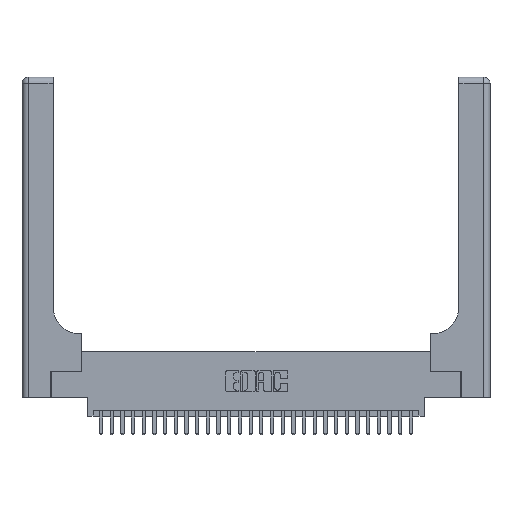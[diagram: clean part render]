
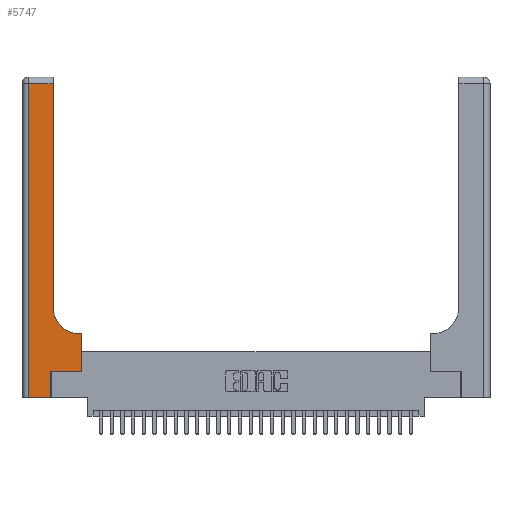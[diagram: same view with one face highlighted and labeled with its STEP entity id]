
A CAD part, top view. The second image highlights one B-rep face of the part: STEP entity #5747.
In plain terms, the highlighted planar face has unit normal (0, 0, 1).
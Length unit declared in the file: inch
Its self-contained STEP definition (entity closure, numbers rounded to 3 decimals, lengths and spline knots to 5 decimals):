
#76 = FACE_OUTER_BOUND ( 'NONE', #607, .T. ) ;
#607 = EDGE_LOOP ( 'NONE', ( #3816, #5903, #7704, #10408, #11895, #14027, #17095, #24863, #25956 ) ) ;
#876 = LINE ( 'NONE', #13336, #19120 ) ;
#1017 = CARTESIAN_POINT ( 'NONE',  ( 0.2915, 0.6, 0.37 ) ) ;
#1021 = CARTESIAN_POINT ( 'NONE',  ( 0.5415, 0.85, 0.37 ) ) ;
#1542 = LINE ( 'NONE', #1017, #4173 ) ;
#2059 = CARTESIAN_POINT ( 'NONE',  ( 0.5585, 0.6, 0.37 ) ) ;
#2779 = CARTESIAN_POINT ( 'NONE',  ( 0., 3., 0.37 ) ) ;
#3364 = LINE ( 'NONE', #28676, #16744 ) ;
#3437 = DIRECTION ( 'NONE',  ( 1., 0., 0. ) ) ;
#3473 = EDGE_CURVE ( 'NONE', #10679, #6550, #18507, .T. ) ;
#3590 = VERTEX_POINT ( 'NONE', #25736 ) ;
#3816 = ORIENTED_EDGE ( 'NONE', *, *, #27646, .T. ) ;
#4173 = VECTOR ( 'NONE', #24649, 39.37008 ) ;
#4844 = DIRECTION ( 'NONE',  ( -1., 0., 0. ) ) ;
#5107 = VECTOR ( 'NONE', #30121, 39.37008 ) ;
#5191 = DIRECTION ( 'NONE',  ( 0., 0., -1. ) ) ;
#5558 = VERTEX_POINT ( 'NONE', #2059 ) ;
#5747 = ADVANCED_FACE ( 'NONE', ( #76 ), #17042, .F. ) ;
#5893 = CARTESIAN_POINT ( 'NONE',  ( 0.06, 3., 0.37 ) ) ;
#5903 = ORIENTED_EDGE ( 'NONE', *, *, #14313, .T. ) ;
#6550 = VERTEX_POINT ( 'NONE', #22032 ) ;
#7219 = CARTESIAN_POINT ( 'NONE',  ( 0., 2.94, 0.37 ) ) ;
#7704 = ORIENTED_EDGE ( 'NONE', *, *, #7929, .T. ) ;
#7929 = EDGE_CURVE ( 'NONE', #3590, #10679, #9997, .T. ) ;
#8371 = LINE ( 'NONE', #11096, #13962 ) ;
#8708 = DIRECTION ( 'NONE',  ( 0., 1., 0. ) ) ;
#8844 = VERTEX_POINT ( 'NONE', #20648 ) ;
#9689 = VERTEX_POINT ( 'NONE', #12476 ) ;
#9997 = LINE ( 'NONE', #5893, #17112 ) ;
#10406 = VECTOR ( 'NONE', #26444, 39.37008 ) ;
#10408 = ORIENTED_EDGE ( 'NONE', *, *, #3473, .T. ) ;
#10679 = VERTEX_POINT ( 'NONE', #15997 ) ;
#10948 = DIRECTION ( 'NONE',  ( 1., 0., 0. ) ) ;
#11096 = CARTESIAN_POINT ( 'NONE',  ( 0.5585, 0.25, 0.37 ) ) ;
#11895 = ORIENTED_EDGE ( 'NONE', *, *, #12980, .T. ) ;
#12476 = CARTESIAN_POINT ( 'NONE',  ( 0.269, 0.25, 0.37 ) ) ;
#12980 = EDGE_CURVE ( 'NONE', #6550, #9689, #3364, .T. ) ;
#13336 = CARTESIAN_POINT ( 'NONE',  ( 0.269, 0.25, 0.37 ) ) ;
#13962 = VECTOR ( 'NONE', #8708, 39.37008 ) ;
#14027 = ORIENTED_EDGE ( 'NONE', *, *, #29361, .T. ) ;
#14313 = EDGE_CURVE ( 'NONE', #8844, #3590, #17438, .T. ) ;
#14618 = CARTESIAN_POINT ( 'NONE',  ( 0.2915, 3., 0.37 ) ) ;
#14659 = CARTESIAN_POINT ( 'NONE',  ( 0.5585, 0.25, 0.37 ) ) ;
#15997 = CARTESIAN_POINT ( 'NONE',  ( 0.06, 0., 0.37 ) ) ;
#16744 = VECTOR ( 'NONE', #26422, 39.37008 ) ;
#16760 = LINE ( 'NONE', #14618, #10406 ) ;
#17042 = PLANE ( 'NONE',  #22698 ) ;
#17095 = ORIENTED_EDGE ( 'NONE', *, *, #18172, .T. ) ;
#17112 = VECTOR ( 'NONE', #20122, 39.37008 ) ;
#17438 = LINE ( 'NONE', #7219, #29125 ) ;
#17695 = DIRECTION ( 'NONE',  ( 0., 0., -1. ) ) ;
#18172 = EDGE_CURVE ( 'NONE', #27009, #5558, #8371, .T. ) ;
#18385 = CARTESIAN_POINT ( 'NONE',  ( 0., 0., 0.37 ) ) ;
#18507 = LINE ( 'NONE', #18385, #5107 ) ;
#18672 = VERTEX_POINT ( 'NONE', #20032 ) ;
#19120 = VECTOR ( 'NONE', #10948, 39.37008 ) ;
#20032 = CARTESIAN_POINT ( 'NONE',  ( 0.2915, 0.85, 0.37 ) ) ;
#20122 = DIRECTION ( 'NONE',  ( 0., -1., 0. ) ) ;
#20648 = CARTESIAN_POINT ( 'NONE',  ( 0.2915, 2.94, 0.37 ) ) ;
#21750 = DIRECTION ( 'NONE',  ( -1., 0., 0. ) ) ;
#22032 = CARTESIAN_POINT ( 'NONE',  ( 0.269, 0., 0.37 ) ) ;
#22698 = AXIS2_PLACEMENT_3D ( 'NONE', #2779, #5191, #21750 ) ;
#23832 = AXIS2_PLACEMENT_3D ( 'NONE', #1021, #17695, #3437 ) ;
#24396 = EDGE_CURVE ( 'NONE', #25843, #18672, #28303, .T. ) ;
#24649 = DIRECTION ( 'NONE',  ( -1., 0., 0. ) ) ;
#24863 = ORIENTED_EDGE ( 'NONE', *, *, #27191, .T. ) ;
#25736 = CARTESIAN_POINT ( 'NONE',  ( 0.06, 2.94, 0.37 ) ) ;
#25843 = VERTEX_POINT ( 'NONE', #27519 ) ;
#25956 = ORIENTED_EDGE ( 'NONE', *, *, #24396, .T. ) ;
#26422 = DIRECTION ( 'NONE',  ( 0., 1., 0. ) ) ;
#26444 = DIRECTION ( 'NONE',  ( 0., 1., 0. ) ) ;
#27009 = VERTEX_POINT ( 'NONE', #14659 ) ;
#27191 = EDGE_CURVE ( 'NONE', #5558, #25843, #1542, .T. ) ;
#27519 = CARTESIAN_POINT ( 'NONE',  ( 0.5415, 0.6, 0.37 ) ) ;
#27646 = EDGE_CURVE ( 'NONE', #18672, #8844, #16760, .T. ) ;
#28303 = CIRCLE ( 'NONE', #23832, 0.25 ) ;
#28676 = CARTESIAN_POINT ( 'NONE',  ( 0.269, 0., 0.37 ) ) ;
#29125 = VECTOR ( 'NONE', #4844, 39.37008 ) ;
#29361 = EDGE_CURVE ( 'NONE', #9689, #27009, #876, .T. ) ;
#30121 = DIRECTION ( 'NONE',  ( 1., 0., 0. ) ) ;
